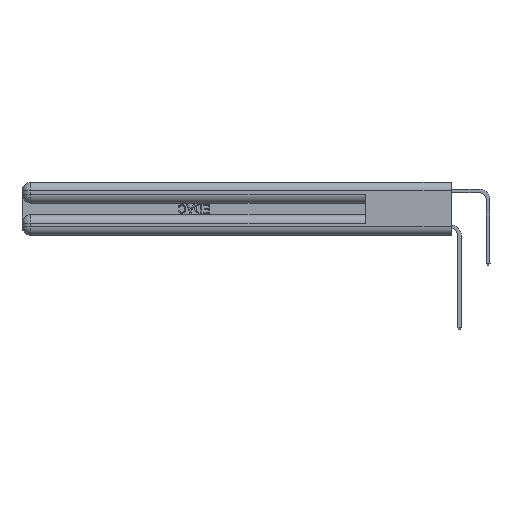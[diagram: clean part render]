
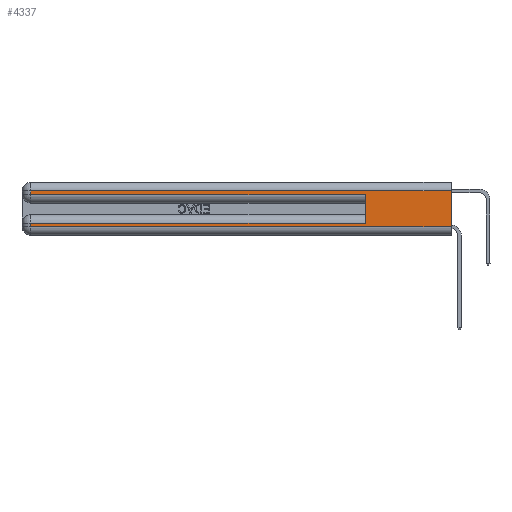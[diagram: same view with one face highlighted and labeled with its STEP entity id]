
A CAD part, left-side view. The second image highlights one B-rep face of the part: STEP entity #4337.
In plain terms, the highlighted planar face has unit normal (-1, 0, 0).
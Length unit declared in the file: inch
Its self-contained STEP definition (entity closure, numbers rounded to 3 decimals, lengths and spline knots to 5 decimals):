
#478 = DIRECTION ( 'NONE',  ( 0., 1., 0. ) ) ;
#1566 = CARTESIAN_POINT ( 'NONE',  ( 0., 0., 0.085 ) ) ;
#2645 = AXIS2_PLACEMENT_3D ( 'NONE', #16837, #14579, #24261 ) ;
#3174 = LINE ( 'NONE', #9055, #8186 ) ;
#3250 = ORIENTED_EDGE ( 'NONE', *, *, #22780, .T. ) ;
#3753 = CARTESIAN_POINT ( 'NONE',  ( 0., 0.6, 0.145 ) ) ;
#4088 = DIRECTION ( 'NONE',  ( 0., 1., 0. ) ) ;
#4132 = EDGE_CURVE ( 'NONE', #13686, #12781, #26493, .T. ) ;
#4215 = VERTEX_POINT ( 'NONE', #7545 ) ;
#4337 = ADVANCED_FACE ( 'NONE', ( #5721 ), #26833, .F. ) ;
#4398 = CARTESIAN_POINT ( 'NONE',  ( 0., 0., 0.06 ) ) ;
#4987 = DIRECTION ( 'NONE',  ( 0., 0., -1. ) ) ;
#5259 = EDGE_CURVE ( 'NONE', #5644, #30741, #6822, .T. ) ;
#5644 = VERTEX_POINT ( 'NONE', #27117 ) ;
#5721 = FACE_OUTER_BOUND ( 'NONE', #8180, .T. ) ;
#6822 = LINE ( 'NONE', #16206, #15649 ) ;
#7545 = CARTESIAN_POINT ( 'NONE',  ( 0., 0., 0.31 ) ) ;
#7725 = LINE ( 'NONE', #3753, #28836 ) ;
#8180 = EDGE_LOOP ( 'NONE', ( #8209, #3250, #25428, #15111, #27906, #17466, #24458, #10103 ) ) ;
#8186 = VECTOR ( 'NONE', #28994, 39.37008 ) ;
#8209 = ORIENTED_EDGE ( 'NONE', *, *, #17537, .F. ) ;
#8576 = CARTESIAN_POINT ( 'NONE',  ( 0., 0.6, 0.285 ) ) ;
#9055 = CARTESIAN_POINT ( 'NONE',  ( 0., 0., 0.285 ) ) ;
#10103 = ORIENTED_EDGE ( 'NONE', *, *, #5259, .T. ) ;
#12781 = VERTEX_POINT ( 'NONE', #15066 ) ;
#13018 = DIRECTION ( 'NONE',  ( 0., 0., -1. ) ) ;
#13404 = CARTESIAN_POINT ( 'NONE',  ( 0., 0.6, 0.085 ) ) ;
#13686 = VERTEX_POINT ( 'NONE', #13404 ) ;
#14089 = EDGE_CURVE ( 'NONE', #24728, #27775, #14589, .T. ) ;
#14579 = DIRECTION ( 'NONE',  ( 1., 0., 0. ) ) ;
#14589 = LINE ( 'NONE', #20028, #26892 ) ;
#14960 = VECTOR ( 'NONE', #4088, 39.37008 ) ;
#15066 = CARTESIAN_POINT ( 'NONE',  ( 0., 2.94, 0.085 ) ) ;
#15111 = ORIENTED_EDGE ( 'NONE', *, *, #16398, .T. ) ;
#15240 = CARTESIAN_POINT ( 'NONE',  ( 0., 0., 0.31 ) ) ;
#15649 = VECTOR ( 'NONE', #17256, 39.37008 ) ;
#16206 = CARTESIAN_POINT ( 'NONE',  ( 0., 0., 0.06 ) ) ;
#16398 = EDGE_CURVE ( 'NONE', #27775, #20020, #3174, .T. ) ;
#16837 = CARTESIAN_POINT ( 'NONE',  ( 0., 0., 0.37 ) ) ;
#17256 = DIRECTION ( 'NONE',  ( 0., -1., 0. ) ) ;
#17466 = ORIENTED_EDGE ( 'NONE', *, *, #4132, .T. ) ;
#17537 = EDGE_CURVE ( 'NONE', #4215, #30741, #24287, .T. ) ;
#19689 = CARTESIAN_POINT ( 'NONE',  ( 0., 0., 0.37 ) ) ;
#20020 = VERTEX_POINT ( 'NONE', #8576 ) ;
#20028 = CARTESIAN_POINT ( 'NONE',  ( 0., 2.94, 0.37 ) ) ;
#20939 = VECTOR ( 'NONE', #478, 39.37008 ) ;
#22780 = EDGE_CURVE ( 'NONE', #4215, #24728, #31620, .T. ) ;
#22815 = CARTESIAN_POINT ( 'NONE',  ( 0., 2.94, 0.37 ) ) ;
#24261 = DIRECTION ( 'NONE',  ( 0., 0., -1. ) ) ;
#24287 = LINE ( 'NONE', #19689, #29246 ) ;
#24458 = ORIENTED_EDGE ( 'NONE', *, *, #27521, .T. ) ;
#24728 = VERTEX_POINT ( 'NONE', #31543 ) ;
#25274 = LINE ( 'NONE', #22815, #25657 ) ;
#25428 = ORIENTED_EDGE ( 'NONE', *, *, #14089, .T. ) ;
#25657 = VECTOR ( 'NONE', #13018, 39.37008 ) ;
#26493 = LINE ( 'NONE', #1566, #14960 ) ;
#26833 = PLANE ( 'NONE',  #2645 ) ;
#26892 = VECTOR ( 'NONE', #29736, 39.37008 ) ;
#27117 = CARTESIAN_POINT ( 'NONE',  ( 0., 2.94, 0.06 ) ) ;
#27521 = EDGE_CURVE ( 'NONE', #12781, #5644, #25274, .T. ) ;
#27775 = VERTEX_POINT ( 'NONE', #28359 ) ;
#27906 = ORIENTED_EDGE ( 'NONE', *, *, #30721, .F. ) ;
#28359 = CARTESIAN_POINT ( 'NONE',  ( 0., 2.94, 0.285 ) ) ;
#28836 = VECTOR ( 'NONE', #28959, 39.37008 ) ;
#28959 = DIRECTION ( 'NONE',  ( 0., 0., 1. ) ) ;
#28994 = DIRECTION ( 'NONE',  ( 0., -1., 0. ) ) ;
#29246 = VECTOR ( 'NONE', #4987, 39.37008 ) ;
#29736 = DIRECTION ( 'NONE',  ( 0., 0., -1. ) ) ;
#30721 = EDGE_CURVE ( 'NONE', #13686, #20020, #7725, .T. ) ;
#30741 = VERTEX_POINT ( 'NONE', #4398 ) ;
#31543 = CARTESIAN_POINT ( 'NONE',  ( 0., 2.94, 0.31 ) ) ;
#31620 = LINE ( 'NONE', #15240, #20939 ) ;
